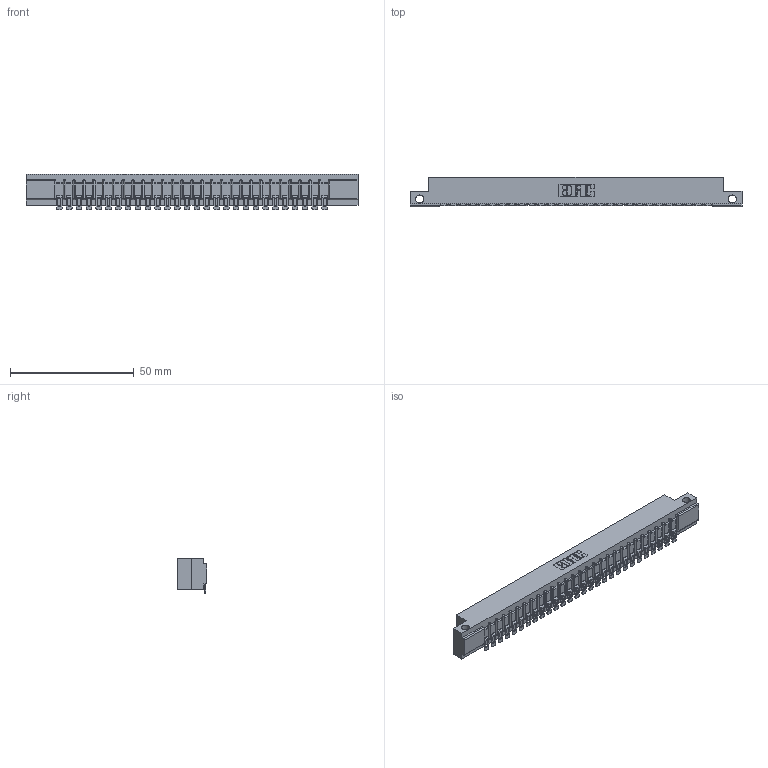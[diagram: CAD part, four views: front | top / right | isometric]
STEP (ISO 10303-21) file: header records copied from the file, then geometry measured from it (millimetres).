
FILE_DESCRIPTION (( 'STEP AP203' ), '1' );
FILE_NAME ('307-028-454-112.STEP', '2020-09-28T07:53:26', ( '' ), ( '' ), 'SwSTEP 2.0', 'SolidWorks 2020', '' );
FILE_SCHEMA (( 'CONFIG_CONTROL_DESIGN' ));
Length unit declared in the file: inch
Products named in the file (3): 307 Part_.128 Dia Side Mounting Holes; 307-290-002_554; 307-028-454-112
Assembly tree (29 placements, depth 2):
  307-028-454-112
    307 Part_.128 Dia Side Mounting Holes
    307-290-002_554  x28
Bounding box: 133.96 x 12.01 x 14.52 mm (x, y, z)
Volume: 14098.9 mm3; surface area: 17517.9 mm2
Topology: 29 solids, 29 shells, 2415 faces, 7407 edges, 4858 vertices
Faces by surface type: plane 1358, cylinder 999, sphere 58
Entity records: 26697 total; most frequent: CARTESIAN_POINT 4502, ORIENTED_EDGE 4492, DIRECTION 4386, EDGE_CURVE 2246, VECTOR 1706, LINE 1706, VERTEX_POINT 1456, AXIS2_PLACEMENT_3D 1340
